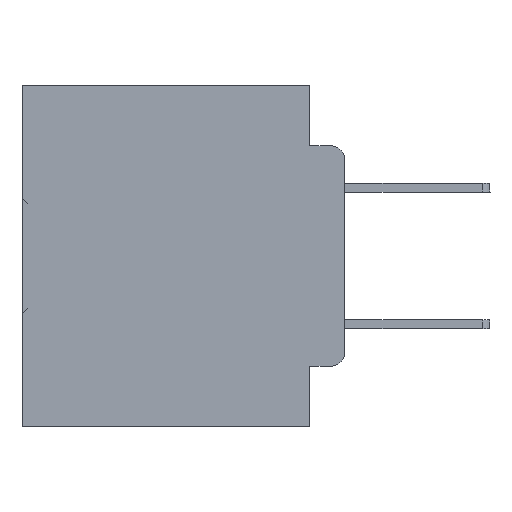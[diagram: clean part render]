
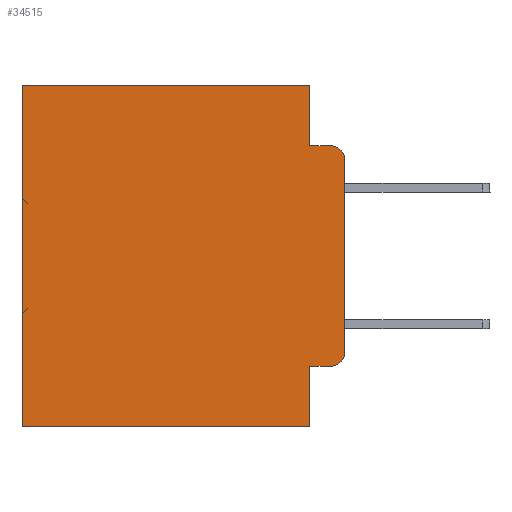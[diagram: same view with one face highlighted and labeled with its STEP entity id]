
A CAD part, left-side view. The second image highlights one B-rep face of the part: STEP entity #34515.
In plain terms, the highlighted planar face has unit normal (-1, 0, 0).
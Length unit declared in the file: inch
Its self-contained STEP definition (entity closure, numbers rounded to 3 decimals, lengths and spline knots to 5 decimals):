
#501 = VERTEX_POINT ( 'NONE', #13727 ) ;
#629 = VECTOR ( 'NONE', #4111, 39.37008 ) ;
#1293 = CARTESIAN_POINT ( 'NONE',  ( 0.298, 0.051, -0.4115 ) ) ;
#1650 = LINE ( 'NONE', #7117, #32168 ) ;
#1938 = CIRCLE ( 'NONE', #36856, 0.02 ) ;
#2338 = EDGE_CURVE ( 'NONE', #14887, #501, #28239, .T. ) ;
#3072 = CARTESIAN_POINT ( 'NONE',  ( 0.298, 0., 0. ) ) ;
#3469 = EDGE_CURVE ( 'NONE', #30491, #8401, #23786, .T. ) ;
#3732 = ORIENTED_EDGE ( 'NONE', *, *, #35872, .F. ) ;
#4111 = DIRECTION ( 'NONE',  ( 0., 1., 0. ) ) ;
#4695 = CARTESIAN_POINT ( 'NONE',  ( 0.298, 0., -0.1085 ) ) ;
#4771 = ORIENTED_EDGE ( 'NONE', *, *, #6210, .F. ) ;
#4901 = CARTESIAN_POINT ( 'NONE',  ( 0.298, 0.051, 0. ) ) ;
#6027 = EDGE_CURVE ( 'NONE', #30491, #17894, #28147, .T. ) ;
#6143 = PLANE ( 'NONE',  #32717 ) ;
#6210 = EDGE_CURVE ( 'NONE', #14887, #18447, #29104, .T. ) ;
#6572 = ORIENTED_EDGE ( 'NONE', *, *, #36297, .T. ) ;
#6675 = DIRECTION ( 'NONE',  ( 0., 0., -1. ) ) ;
#6699 = VERTEX_POINT ( 'NONE', #4695 ) ;
#7117 = CARTESIAN_POINT ( 'NONE',  ( 0.298, 0., 0. ) ) ;
#8401 = VERTEX_POINT ( 'NONE', #18940 ) ;
#8748 = DIRECTION ( 'NONE',  ( 0., -1., 0. ) ) ;
#11869 = DIRECTION ( 'NONE',  ( 0., 1., 0. ) ) ;
#12235 = CARTESIAN_POINT ( 'NONE',  ( 0.298, 0.02, -0.0885 ) ) ;
#12589 = CARTESIAN_POINT ( 'NONE',  ( 0.298, 0.051, 0. ) ) ;
#12762 = ORIENTED_EDGE ( 'NONE', *, *, #19865, .T. ) ;
#13344 = DIRECTION ( 'NONE',  ( 0., 0., -1. ) ) ;
#13727 = CARTESIAN_POINT ( 'NONE',  ( 0.298, 0.02, -0.4115 ) ) ;
#13876 = EDGE_LOOP ( 'NONE', ( #3732, #33460, #34395, #19665, #34593, #12762, #14367, #4771, #34005, #6572 ) ) ;
#14195 = EDGE_CURVE ( 'NONE', #17894, #16653, #20883, .T. ) ;
#14367 = ORIENTED_EDGE ( 'NONE', *, *, #18944, .F. ) ;
#14887 = VERTEX_POINT ( 'NONE', #24953 ) ;
#15335 = CARTESIAN_POINT ( 'NONE',  ( 0.298, 0., 0. ) ) ;
#15725 = FACE_OUTER_BOUND ( 'NONE', #13876, .T. ) ;
#16256 = DIRECTION ( 'NONE',  ( -1., 0., 0. ) ) ;
#16653 = VERTEX_POINT ( 'NONE', #12235 ) ;
#16823 = DIRECTION ( 'NONE',  ( 0., 0., -1. ) ) ;
#17894 = VERTEX_POINT ( 'NONE', #36418 ) ;
#18447 = VERTEX_POINT ( 'NONE', #34209 ) ;
#18642 = VECTOR ( 'NONE', #16823, 39.37008 ) ;
#18738 = VECTOR ( 'NONE', #11869, 39.37008 ) ;
#18830 = EDGE_CURVE ( 'NONE', #6699, #16653, #29307, .T. ) ;
#18940 = CARTESIAN_POINT ( 'NONE',  ( 0.298, 0.473, 0. ) ) ;
#18944 = EDGE_CURVE ( 'NONE', #18447, #24914, #25604, .T. ) ;
#19665 = ORIENTED_EDGE ( 'NONE', *, *, #6027, .F. ) ;
#19865 = EDGE_CURVE ( 'NONE', #8401, #24914, #37135, .T. ) ;
#20883 = LINE ( 'NONE', #35501, #21051 ) ;
#21051 = VECTOR ( 'NONE', #8748, 39.37008 ) ;
#22098 = DIRECTION ( 'NONE',  ( 0., 0., -1. ) ) ;
#22209 = DIRECTION ( 'NONE',  ( 0., -1., 0. ) ) ;
#22364 = DIRECTION ( 'NONE',  ( 0., 0., -1. ) ) ;
#23786 = LINE ( 'NONE', #3072, #18738 ) ;
#24822 = CARTESIAN_POINT ( 'NONE',  ( 0.298, 0., -0.5 ) ) ;
#24914 = VERTEX_POINT ( 'NONE', #28510 ) ;
#24953 = CARTESIAN_POINT ( 'NONE',  ( 0.298, 0.051, -0.4115 ) ) ;
#25240 = CARTESIAN_POINT ( 'NONE',  ( 0.298, 0.051, 0. ) ) ;
#25407 = CARTESIAN_POINT ( 'NONE',  ( 0.298, 0.02, -0.1085 ) ) ;
#25604 = LINE ( 'NONE', #24822, #629 ) ;
#27575 = CARTESIAN_POINT ( 'NONE',  ( 0.298, 0.02, -0.3915 ) ) ;
#28147 = LINE ( 'NONE', #25240, #31009 ) ;
#28239 = LINE ( 'NONE', #1293, #34886 ) ;
#28510 = CARTESIAN_POINT ( 'NONE',  ( 0.298, 0.473, -0.5 ) ) ;
#28731 = CARTESIAN_POINT ( 'NONE',  ( 0.298, 0.473, 0. ) ) ;
#29104 = LINE ( 'NONE', #4901, #18642 ) ;
#29307 = CIRCLE ( 'NONE', #34287, 0.02 ) ;
#29713 = CARTESIAN_POINT ( 'NONE',  ( 0.298, 0., -0.3915 ) ) ;
#29950 = DIRECTION ( 'NONE',  ( 0., 0., -1. ) ) ;
#30491 = VERTEX_POINT ( 'NONE', #12589 ) ;
#30770 = VERTEX_POINT ( 'NONE', #29713 ) ;
#31009 = VECTOR ( 'NONE', #6675, 39.37008 ) ;
#31237 = DIRECTION ( 'NONE',  ( -1., 0., 0. ) ) ;
#32168 = VECTOR ( 'NONE', #22364, 39.37008 ) ;
#32717 = AXIS2_PLACEMENT_3D ( 'NONE', #15335, #33456, #29950 ) ;
#33456 = DIRECTION ( 'NONE',  ( 1., 0., 0. ) ) ;
#33460 = ORIENTED_EDGE ( 'NONE', *, *, #18830, .T. ) ;
#34005 = ORIENTED_EDGE ( 'NONE', *, *, #2338, .T. ) ;
#34195 = DIRECTION ( 'NONE',  ( 0., 0., -1. ) ) ;
#34209 = CARTESIAN_POINT ( 'NONE',  ( 0.298, 0.051, -0.5 ) ) ;
#34287 = AXIS2_PLACEMENT_3D ( 'NONE', #25407, #31237, #22098 ) ;
#34395 = ORIENTED_EDGE ( 'NONE', *, *, #14195, .F. ) ;
#34515 = ADVANCED_FACE ( 'NONE', ( #15725 ), #6143, .F. ) ;
#34593 = ORIENTED_EDGE ( 'NONE', *, *, #3469, .T. ) ;
#34886 = VECTOR ( 'NONE', #22209, 39.37008 ) ;
#35501 = CARTESIAN_POINT ( 'NONE',  ( 0.298, 0.051, -0.0885 ) ) ;
#35594 = VECTOR ( 'NONE', #34195, 39.37008 ) ;
#35872 = EDGE_CURVE ( 'NONE', #6699, #30770, #1650, .T. ) ;
#36297 = EDGE_CURVE ( 'NONE', #501, #30770, #1938, .T. ) ;
#36418 = CARTESIAN_POINT ( 'NONE',  ( 0.298, 0.051, -0.0885 ) ) ;
#36856 = AXIS2_PLACEMENT_3D ( 'NONE', #27575, #16256, #13344 ) ;
#37135 = LINE ( 'NONE', #28731, #35594 ) ;
